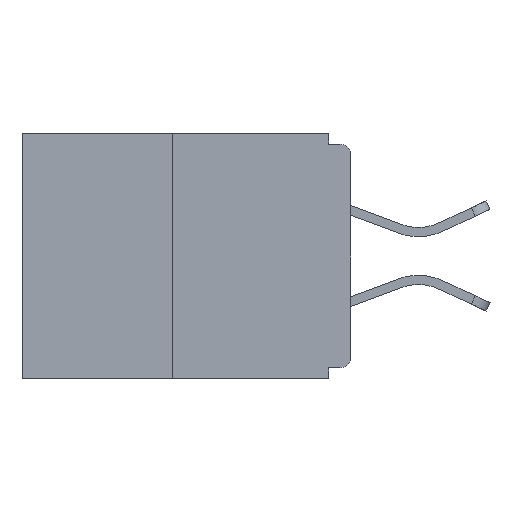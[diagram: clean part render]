
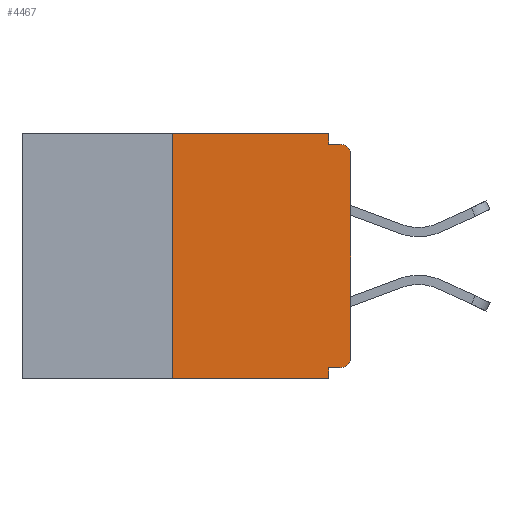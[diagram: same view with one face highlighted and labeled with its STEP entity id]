
A CAD part, left-side view. The second image highlights one B-rep face of the part: STEP entity #4467.
In plain terms, the highlighted planar face has unit normal (-1, 0, 0).
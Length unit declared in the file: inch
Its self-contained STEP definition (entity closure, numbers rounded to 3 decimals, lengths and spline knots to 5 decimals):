
#326 = DIRECTION ( 'NONE',  ( 0., 0., -1. ) ) ;
#541 = ORIENTED_EDGE ( 'NONE', *, *, #24661, .F. ) ;
#566 = ORIENTED_EDGE ( 'NONE', *, *, #8925, .T. ) ;
#1448 = ORIENTED_EDGE ( 'NONE', *, *, #24514, .T. ) ;
#1864 = CIRCLE ( 'NONE', #6846, 0.015 ) ;
#2093 = DIRECTION ( 'NONE',  ( 0., 1., 0. ) ) ;
#2198 = EDGE_CURVE ( 'NONE', #22396, #7579, #10049, .T. ) ;
#2612 = DIRECTION ( 'NONE',  ( 0., 0., -1. ) ) ;
#3006 = LINE ( 'NONE', #21951, #18112 ) ;
#4018 = CARTESIAN_POINT ( 'NONE',  ( 0., 0.015, -0.015 ) ) ;
#4046 = VERTEX_POINT ( 'NONE', #12985 ) ;
#4284 = LINE ( 'NONE', #16245, #16013 ) ;
#4467 = ADVANCED_FACE ( 'NONE', ( #20839 ), #8896, .F. ) ;
#4871 = VECTOR ( 'NONE', #29023, 39.37008 ) ;
#5623 = DIRECTION ( 'NONE',  ( 0., 0., 1. ) ) ;
#5960 = CARTESIAN_POINT ( 'NONE',  ( 0., 0., -0.03 ) ) ;
#6325 = VECTOR ( 'NONE', #18609, 39.37008 ) ;
#6839 = LINE ( 'NONE', #30009, #6325 ) ;
#6846 = AXIS2_PLACEMENT_3D ( 'NONE', #12451, #13036, #17706 ) ;
#7490 = CARTESIAN_POINT ( 'NONE',  ( 0., 0.031, 0. ) ) ;
#7529 = DIRECTION ( 'NONE',  ( -1., 0., 0. ) ) ;
#7579 = VERTEX_POINT ( 'NONE', #13294 ) ;
#8787 = ORIENTED_EDGE ( 'NONE', *, *, #2198, .F. ) ;
#8896 = PLANE ( 'NONE',  #11105 ) ;
#8925 = EDGE_CURVE ( 'NONE', #12819, #7579, #26037, .T. ) ;
#9098 = CARTESIAN_POINT ( 'NONE',  ( 0., 0.031, -0.328 ) ) ;
#9710 = EDGE_CURVE ( 'NONE', #13823, #23070, #12333, .T. ) ;
#10049 = LINE ( 'NONE', #28763, #11226 ) ;
#10175 = VECTOR ( 'NONE', #14754, 39.37008 ) ;
#11038 = LINE ( 'NONE', #22560, #30297 ) ;
#11105 = AXIS2_PLACEMENT_3D ( 'NONE', #28015, #15865, #20223 ) ;
#11226 = VECTOR ( 'NONE', #2612, 39.37008 ) ;
#12208 = CARTESIAN_POINT ( 'NONE',  ( 0., 0.46, -0.343 ) ) ;
#12333 = CIRCLE ( 'NONE', #25734, 0.015 ) ;
#12451 = CARTESIAN_POINT ( 'NONE',  ( 0., 0.015, -0.313 ) ) ;
#12819 = VERTEX_POINT ( 'NONE', #26777 ) ;
#12985 = CARTESIAN_POINT ( 'NONE',  ( 0., 0.015, -0.328 ) ) ;
#13036 = DIRECTION ( 'NONE',  ( -1., 0., 0. ) ) ;
#13232 = DIRECTION ( 'NONE',  ( 0., 0., 1. ) ) ;
#13294 = CARTESIAN_POINT ( 'NONE',  ( 0., 0.031, -0.343 ) ) ;
#13366 = VERTEX_POINT ( 'NONE', #28238 ) ;
#13823 = VERTEX_POINT ( 'NONE', #5960 ) ;
#14294 = LINE ( 'NONE', #23620, #10175 ) ;
#14477 = EDGE_CURVE ( 'NONE', #22303, #23070, #14294, .T. ) ;
#14754 = DIRECTION ( 'NONE',  ( 0., -1., 0. ) ) ;
#15113 = ORIENTED_EDGE ( 'NONE', *, *, #18986, .T. ) ;
#15865 = DIRECTION ( 'NONE',  ( 1., 0., 0. ) ) ;
#16013 = VECTOR ( 'NONE', #2093, 39.37008 ) ;
#16245 = CARTESIAN_POINT ( 'NONE',  ( 0., 0., -0.328 ) ) ;
#16936 = ORIENTED_EDGE ( 'NONE', *, *, #22315, .F. ) ;
#17706 = DIRECTION ( 'NONE',  ( 0., 0., -1. ) ) ;
#18112 = VECTOR ( 'NONE', #5623, 39.37008 ) ;
#18609 = DIRECTION ( 'NONE',  ( 0., -1., 0. ) ) ;
#18810 = EDGE_LOOP ( 'NONE', ( #26704, #29801, #566, #8787, #16936, #15113, #1448, #25661, #22185, #541 ) ) ;
#18986 = EDGE_CURVE ( 'NONE', #4046, #13366, #1864, .T. ) ;
#19622 = DIRECTION ( 'NONE',  ( 0., 0., -1. ) ) ;
#20223 = DIRECTION ( 'NONE',  ( 0., 0., -1. ) ) ;
#20839 = FACE_OUTER_BOUND ( 'NONE', #18810, .T. ) ;
#21192 = EDGE_CURVE ( 'NONE', #12819, #30294, #11038, .T. ) ;
#21951 = CARTESIAN_POINT ( 'NONE',  ( 0., 0., 0. ) ) ;
#22185 = ORIENTED_EDGE ( 'NONE', *, *, #14477, .F. ) ;
#22303 = VERTEX_POINT ( 'NONE', #22621 ) ;
#22315 = EDGE_CURVE ( 'NONE', #4046, #22396, #4284, .T. ) ;
#22396 = VERTEX_POINT ( 'NONE', #9098 ) ;
#22560 = CARTESIAN_POINT ( 'NONE',  ( 0., 0.25, 0. ) ) ;
#22621 = CARTESIAN_POINT ( 'NONE',  ( 0., 0.031, -0.015 ) ) ;
#23070 = VERTEX_POINT ( 'NONE', #4018 ) ;
#23086 = VECTOR ( 'NONE', #326, 39.37008 ) ;
#23326 = CARTESIAN_POINT ( 'NONE',  ( 0., 0.031, 0. ) ) ;
#23620 = CARTESIAN_POINT ( 'NONE',  ( 0., 0., -0.015 ) ) ;
#23638 = LINE ( 'NONE', #7490, #23086 ) ;
#24514 = EDGE_CURVE ( 'NONE', #13366, #13823, #3006, .T. ) ;
#24661 = EDGE_CURVE ( 'NONE', #28277, #22303, #23638, .T. ) ;
#25661 = ORIENTED_EDGE ( 'NONE', *, *, #9710, .T. ) ;
#25734 = AXIS2_PLACEMENT_3D ( 'NONE', #28851, #7529, #19622 ) ;
#26037 = LINE ( 'NONE', #12208, #4871 ) ;
#26300 = EDGE_CURVE ( 'NONE', #30294, #28277, #6839, .T. ) ;
#26704 = ORIENTED_EDGE ( 'NONE', *, *, #26300, .F. ) ;
#26777 = CARTESIAN_POINT ( 'NONE',  ( 0., 0.25, -0.343 ) ) ;
#28015 = CARTESIAN_POINT ( 'NONE',  ( 0., 0.46, 0. ) ) ;
#28238 = CARTESIAN_POINT ( 'NONE',  ( 0., 0., -0.313 ) ) ;
#28277 = VERTEX_POINT ( 'NONE', #23326 ) ;
#28763 = CARTESIAN_POINT ( 'NONE',  ( 0., 0.031, -0.343 ) ) ;
#28851 = CARTESIAN_POINT ( 'NONE',  ( 0., 0.015, -0.03 ) ) ;
#29023 = DIRECTION ( 'NONE',  ( 0., -1., 0. ) ) ;
#29352 = CARTESIAN_POINT ( 'NONE',  ( 0., 0.25, 0. ) ) ;
#29801 = ORIENTED_EDGE ( 'NONE', *, *, #21192, .F. ) ;
#30009 = CARTESIAN_POINT ( 'NONE',  ( 0., 0.46, 0. ) ) ;
#30294 = VERTEX_POINT ( 'NONE', #29352 ) ;
#30297 = VECTOR ( 'NONE', #13232, 39.37008 ) ;
